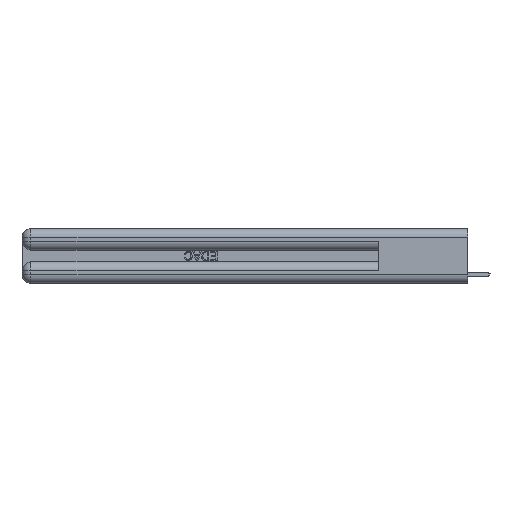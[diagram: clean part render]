
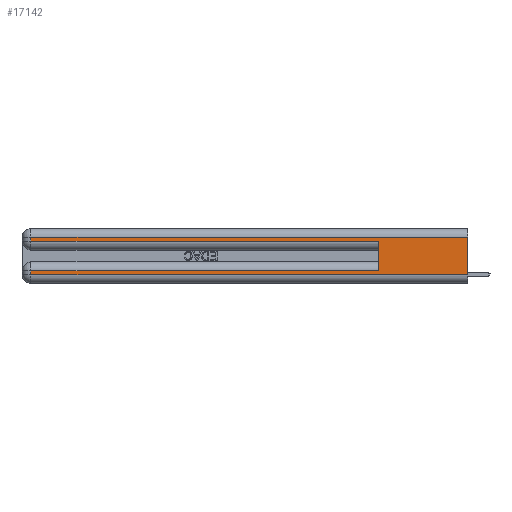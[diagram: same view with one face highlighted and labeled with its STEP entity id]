
A CAD part, left-side view. The second image highlights one B-rep face of the part: STEP entity #17142.
In plain terms, the highlighted planar face has unit normal (-1, 0, 0).
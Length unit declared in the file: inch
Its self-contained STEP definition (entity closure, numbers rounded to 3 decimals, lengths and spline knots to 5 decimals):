
#88 = LINE ( 'NONE', #7668, #2543 ) ;
#463 = LINE ( 'NONE', #2106, #10816 ) ;
#613 = LINE ( 'NONE', #16115, #27386 ) ;
#1569 = ORIENTED_EDGE ( 'NONE', *, *, #1859, .T. ) ;
#1859 = EDGE_CURVE ( 'NONE', #14158, #7150, #23082, .T. ) ;
#2106 = CARTESIAN_POINT ( 'NONE',  ( 0., 0., 0.31 ) ) ;
#2211 = EDGE_CURVE ( 'NONE', #7150, #20742, #7667, .T. ) ;
#2543 = VECTOR ( 'NONE', #2584, 39.37008 ) ;
#2584 = DIRECTION ( 'NONE',  ( 0., 1., 0. ) ) ;
#2923 = CARTESIAN_POINT ( 'NONE',  ( 0., 0.6, 0.285 ) ) ;
#2930 = VECTOR ( 'NONE', #4572, 39.37008 ) ;
#4572 = DIRECTION ( 'NONE',  ( 0., 0., -1. ) ) ;
#4616 = ORIENTED_EDGE ( 'NONE', *, *, #19595, .T. ) ;
#5526 = CARTESIAN_POINT ( 'NONE',  ( 0., 2.94, 0.085 ) ) ;
#5708 = DIRECTION ( 'NONE',  ( 1., 0., 0. ) ) ;
#5943 = VECTOR ( 'NONE', #20178, 39.37008 ) ;
#6152 = CARTESIAN_POINT ( 'NONE',  ( 0., 2.94, 0.285 ) ) ;
#6211 = ORIENTED_EDGE ( 'NONE', *, *, #14945, .F. ) ;
#6357 = DIRECTION ( 'NONE',  ( 0., -1., 0. ) ) ;
#6734 = ORIENTED_EDGE ( 'NONE', *, *, #15041, .T. ) ;
#7150 = VERTEX_POINT ( 'NONE', #6152 ) ;
#7667 = LINE ( 'NONE', #19400, #24791 ) ;
#7668 = CARTESIAN_POINT ( 'NONE',  ( 0., 0., 0.085 ) ) ;
#8038 = LINE ( 'NONE', #17101, #20648 ) ;
#8728 = VERTEX_POINT ( 'NONE', #9009 ) ;
#9009 = CARTESIAN_POINT ( 'NONE',  ( 0., 0., 0.06 ) ) ;
#9158 = VERTEX_POINT ( 'NONE', #25303 ) ;
#10291 = DIRECTION ( 'NONE',  ( 0., 0., 1. ) ) ;
#10816 = VECTOR ( 'NONE', #28652, 39.37008 ) ;
#11488 = DIRECTION ( 'NONE',  ( 0., -1., 0. ) ) ;
#12314 = ORIENTED_EDGE ( 'NONE', *, *, #24177, .F. ) ;
#12584 = CARTESIAN_POINT ( 'NONE',  ( 0., 0.6, 0.085 ) ) ;
#13302 = ORIENTED_EDGE ( 'NONE', *, *, #19420, .T. ) ;
#14158 = VERTEX_POINT ( 'NONE', #27306 ) ;
#14297 = CARTESIAN_POINT ( 'NONE',  ( 0., 0., 0.37 ) ) ;
#14402 = LINE ( 'NONE', #27099, #2930 ) ;
#14600 = ORIENTED_EDGE ( 'NONE', *, *, #18818, .T. ) ;
#14609 = DIRECTION ( 'NONE',  ( 0., 0., -1. ) ) ;
#14945 = EDGE_CURVE ( 'NONE', #18946, #20742, #8038, .T. ) ;
#15041 = EDGE_CURVE ( 'NONE', #25933, #14158, #463, .T. ) ;
#16115 = CARTESIAN_POINT ( 'NONE',  ( 0., 0., 0.06 ) ) ;
#16904 = ORIENTED_EDGE ( 'NONE', *, *, #2211, .T. ) ;
#17072 = FACE_OUTER_BOUND ( 'NONE', #17988, .T. ) ;
#17101 = CARTESIAN_POINT ( 'NONE',  ( 0., 0.6, 0.145 ) ) ;
#17142 = ADVANCED_FACE ( 'NONE', ( #17072 ), #20958, .F. ) ;
#17988 = EDGE_LOOP ( 'NONE', ( #12314, #6734, #1569, #16904, #6211, #13302, #4616, #14600 ) ) ;
#18590 = LINE ( 'NONE', #27981, #19624 ) ;
#18818 = EDGE_CURVE ( 'NONE', #9158, #8728, #613, .T. ) ;
#18946 = VERTEX_POINT ( 'NONE', #12584 ) ;
#19400 = CARTESIAN_POINT ( 'NONE',  ( 0., 0., 0.285 ) ) ;
#19420 = EDGE_CURVE ( 'NONE', #18946, #26142, #88, .T. ) ;
#19595 = EDGE_CURVE ( 'NONE', #26142, #9158, #18590, .T. ) ;
#19624 = VECTOR ( 'NONE', #14609, 39.37008 ) ;
#20178 = DIRECTION ( 'NONE',  ( 0., 0., -1. ) ) ;
#20648 = VECTOR ( 'NONE', #10291, 39.37008 ) ;
#20742 = VERTEX_POINT ( 'NONE', #2923 ) ;
#20958 = PLANE ( 'NONE',  #27343 ) ;
#23082 = LINE ( 'NONE', #24931, #5943 ) ;
#24177 = EDGE_CURVE ( 'NONE', #25933, #8728, #14402, .T. ) ;
#24791 = VECTOR ( 'NONE', #6357, 39.37008 ) ;
#24931 = CARTESIAN_POINT ( 'NONE',  ( 0., 2.94, 0.37 ) ) ;
#25303 = CARTESIAN_POINT ( 'NONE',  ( 0., 2.94, 0.06 ) ) ;
#25737 = DIRECTION ( 'NONE',  ( 0., 0., -1. ) ) ;
#25933 = VERTEX_POINT ( 'NONE', #26708 ) ;
#26142 = VERTEX_POINT ( 'NONE', #5526 ) ;
#26708 = CARTESIAN_POINT ( 'NONE',  ( 0., 0., 0.31 ) ) ;
#27099 = CARTESIAN_POINT ( 'NONE',  ( 0., 0., 0.37 ) ) ;
#27306 = CARTESIAN_POINT ( 'NONE',  ( 0., 2.94, 0.31 ) ) ;
#27343 = AXIS2_PLACEMENT_3D ( 'NONE', #14297, #5708, #25737 ) ;
#27386 = VECTOR ( 'NONE', #11488, 39.37008 ) ;
#27981 = CARTESIAN_POINT ( 'NONE',  ( 0., 2.94, 0.37 ) ) ;
#28652 = DIRECTION ( 'NONE',  ( 0., 1., 0. ) ) ;
